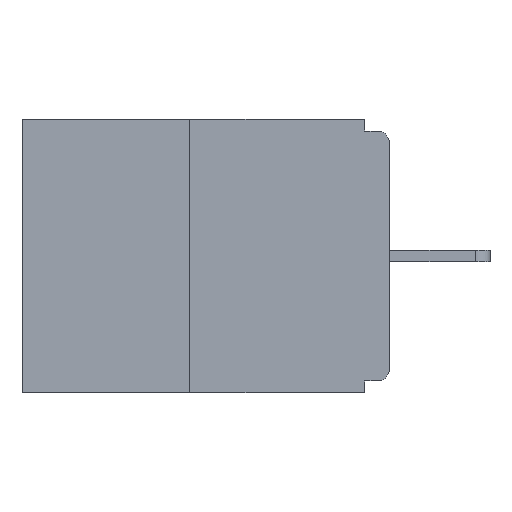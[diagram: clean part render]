
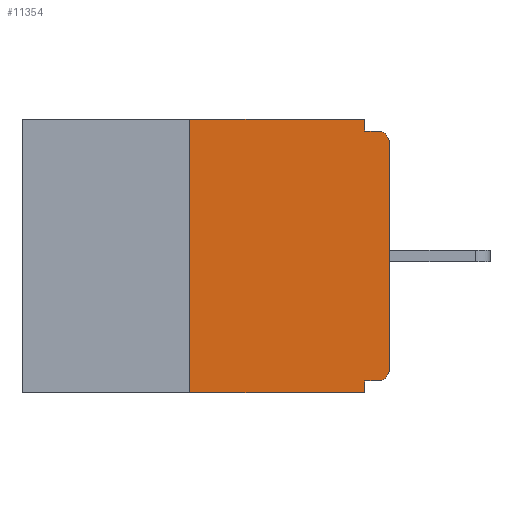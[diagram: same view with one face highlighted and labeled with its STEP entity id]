
A CAD part, left-side view. The second image highlights one B-rep face of the part: STEP entity #11354.
In plain terms, the highlighted planar face has unit normal (-1, 0, 0).
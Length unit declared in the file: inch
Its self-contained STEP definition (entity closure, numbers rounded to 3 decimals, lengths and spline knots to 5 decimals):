
#141 = ORIENTED_EDGE ( 'NONE', *, *, #4840, .F. ) ;
#172 = LINE ( 'NONE', #2665, #12952 ) ;
#280 = LINE ( 'NONE', #4592, #3263 ) ;
#396 = DIRECTION ( 'NONE',  ( 0., 0., -1. ) ) ;
#405 = CARTESIAN_POINT ( 'NONE',  ( 0., 0.25, 0. ) ) ;
#433 = DIRECTION ( 'NONE',  ( -1., 0., 0. ) ) ;
#596 = AXIS2_PLACEMENT_3D ( 'NONE', #6938, #433, #396 ) ;
#605 = VERTEX_POINT ( 'NONE', #2925 ) ;
#705 = AXIS2_PLACEMENT_3D ( 'NONE', #12382, #5109, #13638 ) ;
#891 = VECTOR ( 'NONE', #9049, 39.37008 ) ;
#1292 = LINE ( 'NONE', #6569, #891 ) ;
#1403 = LINE ( 'NONE', #8812, #3954 ) ;
#1655 = ORIENTED_EDGE ( 'NONE', *, *, #11663, .F. ) ;
#1712 = EDGE_CURVE ( 'NONE', #2289, #11175, #1403, .T. ) ;
#1866 = VECTOR ( 'NONE', #6208, 39.37008 ) ;
#2289 = VERTEX_POINT ( 'NONE', #6054 ) ;
#2665 = CARTESIAN_POINT ( 'NONE',  ( 0., 0.031, 0. ) ) ;
#2761 = ORIENTED_EDGE ( 'NONE', *, *, #13154, .F. ) ;
#2925 = CARTESIAN_POINT ( 'NONE',  ( 0., 0., -0.03 ) ) ;
#3063 = ORIENTED_EDGE ( 'NONE', *, *, #14232, .T. ) ;
#3212 = VERTEX_POINT ( 'NONE', #3348 ) ;
#3263 = VECTOR ( 'NONE', #11930, 39.37008 ) ;
#3348 = CARTESIAN_POINT ( 'NONE',  ( 0., 0.031, 0. ) ) ;
#3403 = EDGE_LOOP ( 'NONE', ( #5297, #2761, #4110, #7349, #11065, #12054, #12151, #3063, #1655, #141 ) ) ;
#3424 = VECTOR ( 'NONE', #6899, 39.37008 ) ;
#3777 = CARTESIAN_POINT ( 'NONE',  ( 0., 0., -0.313 ) ) ;
#3853 = PLANE ( 'NONE',  #705 ) ;
#3954 = VECTOR ( 'NONE', #7461, 39.37008 ) ;
#4046 = VERTEX_POINT ( 'NONE', #8542 ) ;
#4110 = ORIENTED_EDGE ( 'NONE', *, *, #9741, .T. ) ;
#4592 = CARTESIAN_POINT ( 'NONE',  ( 0., 0.46, 0. ) ) ;
#4710 = DIRECTION ( 'NONE',  ( -1., 0., 0. ) ) ;
#4791 = LINE ( 'NONE', #4947, #1866 ) ;
#4840 = EDGE_CURVE ( 'NONE', #3212, #9185, #172, .T. ) ;
#4894 = VERTEX_POINT ( 'NONE', #3777 ) ;
#4905 = DIRECTION ( 'NONE',  ( 0., -1., 0. ) ) ;
#4947 = CARTESIAN_POINT ( 'NONE',  ( 0., 0., -0.328 ) ) ;
#5096 = CIRCLE ( 'NONE', #596, 0.015 ) ;
#5109 = DIRECTION ( 'NONE',  ( 1., 0., 0. ) ) ;
#5157 = AXIS2_PLACEMENT_3D ( 'NONE', #12049, #4710, #13261 ) ;
#5199 = EDGE_CURVE ( 'NONE', #4046, #4894, #5096, .T. ) ;
#5297 = ORIENTED_EDGE ( 'NONE', *, *, #10520, .F. ) ;
#6054 = CARTESIAN_POINT ( 'NONE',  ( 0., 0.031, -0.328 ) ) ;
#6208 = DIRECTION ( 'NONE',  ( 0., 1., 0. ) ) ;
#6456 = CARTESIAN_POINT ( 'NONE',  ( 0., 0.015, -0.015 ) ) ;
#6569 = CARTESIAN_POINT ( 'NONE',  ( 0., 0., 0. ) ) ;
#6706 = DIRECTION ( 'NONE',  ( 0., 0., -1. ) ) ;
#6899 = DIRECTION ( 'NONE',  ( 0., -1., 0. ) ) ;
#6938 = CARTESIAN_POINT ( 'NONE',  ( 0., 0.015, -0.313 ) ) ;
#7349 = ORIENTED_EDGE ( 'NONE', *, *, #1712, .F. ) ;
#7418 = CARTESIAN_POINT ( 'NONE',  ( 0., 0.25, 0. ) ) ;
#7461 = DIRECTION ( 'NONE',  ( 0., 0., -1. ) ) ;
#8542 = CARTESIAN_POINT ( 'NONE',  ( 0., 0.015, -0.328 ) ) ;
#8724 = LINE ( 'NONE', #11003, #11551 ) ;
#8812 = CARTESIAN_POINT ( 'NONE',  ( 0., 0.031, -0.343 ) ) ;
#9049 = DIRECTION ( 'NONE',  ( 0., 0., 1. ) ) ;
#9185 = VERTEX_POINT ( 'NONE', #11073 ) ;
#9625 = CARTESIAN_POINT ( 'NONE',  ( 0., 0.031, -0.343 ) ) ;
#9741 = EDGE_CURVE ( 'NONE', #14589, #11175, #8724, .T. ) ;
#10253 = EDGE_CURVE ( 'NONE', #4894, #605, #1292, .T. ) ;
#10520 = EDGE_CURVE ( 'NONE', #12158, #3212, #280, .T. ) ;
#10586 = FACE_OUTER_BOUND ( 'NONE', #3403, .T. ) ;
#11003 = CARTESIAN_POINT ( 'NONE',  ( 0., 0.46, -0.343 ) ) ;
#11065 = ORIENTED_EDGE ( 'NONE', *, *, #11287, .F. ) ;
#11073 = CARTESIAN_POINT ( 'NONE',  ( 0., 0.031, -0.015 ) ) ;
#11175 = VERTEX_POINT ( 'NONE', #9625 ) ;
#11287 = EDGE_CURVE ( 'NONE', #4046, #2289, #4791, .T. ) ;
#11354 = ADVANCED_FACE ( 'NONE', ( #10586 ), #3853, .F. ) ;
#11551 = VECTOR ( 'NONE', #4905, 39.37008 ) ;
#11641 = VECTOR ( 'NONE', #12281, 39.37008 ) ;
#11663 = EDGE_CURVE ( 'NONE', #9185, #14377, #15052, .T. ) ;
#11719 = CARTESIAN_POINT ( 'NONE',  ( 0., 0.25, -0.343 ) ) ;
#11930 = DIRECTION ( 'NONE',  ( 0., -1., 0. ) ) ;
#12031 = LINE ( 'NONE', #7418, #11641 ) ;
#12049 = CARTESIAN_POINT ( 'NONE',  ( 0., 0.015, -0.03 ) ) ;
#12054 = ORIENTED_EDGE ( 'NONE', *, *, #5199, .T. ) ;
#12151 = ORIENTED_EDGE ( 'NONE', *, *, #10253, .T. ) ;
#12158 = VERTEX_POINT ( 'NONE', #405 ) ;
#12281 = DIRECTION ( 'NONE',  ( 0., 0., 1. ) ) ;
#12382 = CARTESIAN_POINT ( 'NONE',  ( 0., 0.46, 0. ) ) ;
#12952 = VECTOR ( 'NONE', #6706, 39.37008 ) ;
#13154 = EDGE_CURVE ( 'NONE', #14589, #12158, #12031, .T. ) ;
#13261 = DIRECTION ( 'NONE',  ( 0., 0., -1. ) ) ;
#13638 = DIRECTION ( 'NONE',  ( 0., 0., -1. ) ) ;
#14172 = CARTESIAN_POINT ( 'NONE',  ( 0., 0., -0.015 ) ) ;
#14232 = EDGE_CURVE ( 'NONE', #605, #14377, #14586, .T. ) ;
#14377 = VERTEX_POINT ( 'NONE', #6456 ) ;
#14586 = CIRCLE ( 'NONE', #5157, 0.015 ) ;
#14589 = VERTEX_POINT ( 'NONE', #11719 ) ;
#15052 = LINE ( 'NONE', #14172, #3424 ) ;
